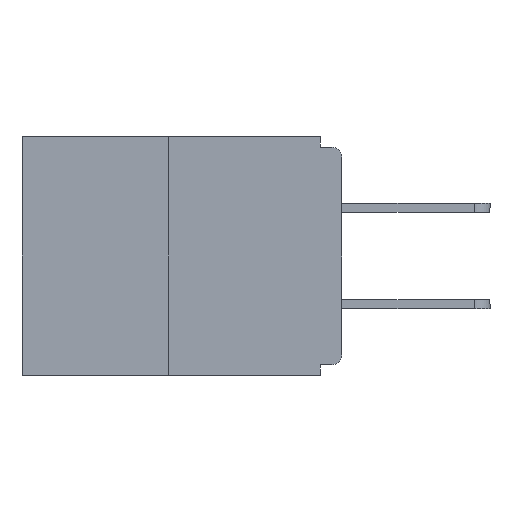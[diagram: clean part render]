
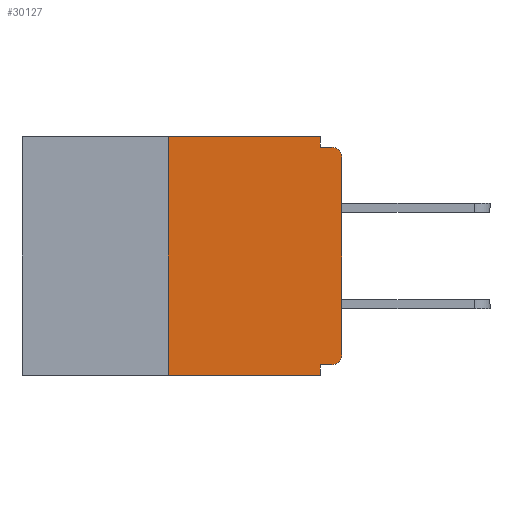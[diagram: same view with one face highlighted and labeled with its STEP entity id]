
A CAD part, left-side view. The second image highlights one B-rep face of the part: STEP entity #30127.
In plain terms, the highlighted planar face has unit normal (-1, 0, 0).
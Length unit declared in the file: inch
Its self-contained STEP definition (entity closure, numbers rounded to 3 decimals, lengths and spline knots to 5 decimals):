
#168 = VECTOR ( 'NONE', #4150, 39.37008 ) ;
#222 = VECTOR ( 'NONE', #31154, 39.37008 ) ;
#537 = CARTESIAN_POINT ( 'NONE',  ( 0., 0.031, -0.328 ) ) ;
#605 = CARTESIAN_POINT ( 'NONE',  ( 0., 0.46, -0.343 ) ) ;
#650 = VECTOR ( 'NONE', #6587, 39.37008 ) ;
#1971 = ORIENTED_EDGE ( 'NONE', *, *, #25293, .F. ) ;
#1997 = LINE ( 'NONE', #8956, #29304 ) ;
#2302 = CARTESIAN_POINT ( 'NONE',  ( 0., 0.031, -0.015 ) ) ;
#2772 = CIRCLE ( 'NONE', #5898, 0.015 ) ;
#2924 = VERTEX_POINT ( 'NONE', #2302 ) ;
#3067 = EDGE_CURVE ( 'NONE', #20193, #16361, #24123, .T. ) ;
#3226 = VERTEX_POINT ( 'NONE', #30207 ) ;
#3488 = DIRECTION ( 'NONE',  ( 0., 0., -1. ) ) ;
#3529 = ORIENTED_EDGE ( 'NONE', *, *, #19720, .F. ) ;
#4104 = CARTESIAN_POINT ( 'NONE',  ( 0., 0.015, -0.015 ) ) ;
#4138 = ORIENTED_EDGE ( 'NONE', *, *, #25420, .F. ) ;
#4150 = DIRECTION ( 'NONE',  ( 0., 0., -1. ) ) ;
#4496 = CARTESIAN_POINT ( 'NONE',  ( 0., 0.25, 0. ) ) ;
#5302 = FACE_OUTER_BOUND ( 'NONE', #24716, .T. ) ;
#5515 = CIRCLE ( 'NONE', #29369, 0.015 ) ;
#5898 = AXIS2_PLACEMENT_3D ( 'NONE', #20658, #10736, #28090 ) ;
#6432 = DIRECTION ( 'NONE',  ( 0., 0., 1. ) ) ;
#6587 = DIRECTION ( 'NONE',  ( 0., 0., 1. ) ) ;
#6754 = CARTESIAN_POINT ( 'NONE',  ( 0., 0.031, 0. ) ) ;
#6783 = DIRECTION ( 'NONE',  ( 1., 0., 0. ) ) ;
#7026 = CARTESIAN_POINT ( 'NONE',  ( 0., 0., 0. ) ) ;
#7106 = LINE ( 'NONE', #7026, #650 ) ;
#7567 = CARTESIAN_POINT ( 'NONE',  ( 0., 0.46, 0. ) ) ;
#7855 = DIRECTION ( 'NONE',  ( 0., -1., 0. ) ) ;
#8956 = CARTESIAN_POINT ( 'NONE',  ( 0., 0.25, 0. ) ) ;
#9000 = CARTESIAN_POINT ( 'NONE',  ( 0., 0.031, -0.343 ) ) ;
#9002 = ORIENTED_EDGE ( 'NONE', *, *, #12672, .F. ) ;
#9441 = CARTESIAN_POINT ( 'NONE',  ( 0., 0., -0.015 ) ) ;
#9682 = ORIENTED_EDGE ( 'NONE', *, *, #10972, .T. ) ;
#10441 = CARTESIAN_POINT ( 'NONE',  ( 0., 0., -0.313 ) ) ;
#10736 = DIRECTION ( 'NONE',  ( -1., 0., 0. ) ) ;
#10972 = EDGE_CURVE ( 'NONE', #27617, #27772, #20453, .T. ) ;
#11623 = DIRECTION ( 'NONE',  ( 0., 0., -1. ) ) ;
#11627 = LINE ( 'NONE', #11649, #30211 ) ;
#11649 = CARTESIAN_POINT ( 'NONE',  ( 0., 0., -0.328 ) ) ;
#11760 = ORIENTED_EDGE ( 'NONE', *, *, #13190, .T. ) ;
#11804 = DIRECTION ( 'NONE',  ( 0., 0., -1. ) ) ;
#12622 = EDGE_CURVE ( 'NONE', #27967, #26005, #7106, .T. ) ;
#12672 = EDGE_CURVE ( 'NONE', #3226, #13007, #11627, .T. ) ;
#13007 = VERTEX_POINT ( 'NONE', #537 ) ;
#13190 = EDGE_CURVE ( 'NONE', #3226, #27967, #5515, .T. ) ;
#14315 = PLANE ( 'NONE',  #19232 ) ;
#15359 = LINE ( 'NONE', #9000, #168 ) ;
#15463 = DIRECTION ( 'NONE',  ( 0., -1., 0. ) ) ;
#15719 = DIRECTION ( 'NONE',  ( -1., 0., 0. ) ) ;
#16305 = CARTESIAN_POINT ( 'NONE',  ( 0., 0., -0.03 ) ) ;
#16361 = VERTEX_POINT ( 'NONE', #20417 ) ;
#16987 = ORIENTED_EDGE ( 'NONE', *, *, #3067, .F. ) ;
#17142 = CARTESIAN_POINT ( 'NONE',  ( 0., 0.031, -0.343 ) ) ;
#17616 = EDGE_CURVE ( 'NONE', #2924, #23178, #30517, .T. ) ;
#18565 = ORIENTED_EDGE ( 'NONE', *, *, #17616, .F. ) ;
#18807 = LINE ( 'NONE', #6754, #19555 ) ;
#19232 = AXIS2_PLACEMENT_3D ( 'NONE', #26232, #6783, #11623 ) ;
#19555 = VECTOR ( 'NONE', #11804, 39.37008 ) ;
#19629 = EDGE_CURVE ( 'NONE', #26005, #23178, #2772, .T. ) ;
#19720 = EDGE_CURVE ( 'NONE', #27617, #20193, #1997, .T. ) ;
#20193 = VERTEX_POINT ( 'NONE', #4496 ) ;
#20360 = CARTESIAN_POINT ( 'NONE',  ( 0., 0.015, -0.313 ) ) ;
#20417 = CARTESIAN_POINT ( 'NONE',  ( 0., 0.031, 0. ) ) ;
#20453 = LINE ( 'NONE', #605, #31016 ) ;
#20658 = CARTESIAN_POINT ( 'NONE',  ( 0., 0.015, -0.03 ) ) ;
#20938 = CARTESIAN_POINT ( 'NONE',  ( 0., 0.25, -0.343 ) ) ;
#22091 = ORIENTED_EDGE ( 'NONE', *, *, #12622, .T. ) ;
#23178 = VERTEX_POINT ( 'NONE', #4104 ) ;
#24123 = LINE ( 'NONE', #7567, #25683 ) ;
#24716 = EDGE_LOOP ( 'NONE', ( #16987, #3529, #9682, #4138, #9002, #11760, #22091, #30137, #18565, #1971 ) ) ;
#25293 = EDGE_CURVE ( 'NONE', #16361, #2924, #18807, .T. ) ;
#25420 = EDGE_CURVE ( 'NONE', #13007, #27772, #15359, .T. ) ;
#25683 = VECTOR ( 'NONE', #7855, 39.37008 ) ;
#26005 = VERTEX_POINT ( 'NONE', #16305 ) ;
#26232 = CARTESIAN_POINT ( 'NONE',  ( 0., 0.46, 0. ) ) ;
#26258 = DIRECTION ( 'NONE',  ( 0., 1., 0. ) ) ;
#27617 = VERTEX_POINT ( 'NONE', #20938 ) ;
#27772 = VERTEX_POINT ( 'NONE', #17142 ) ;
#27967 = VERTEX_POINT ( 'NONE', #10441 ) ;
#28090 = DIRECTION ( 'NONE',  ( 0., 0., -1. ) ) ;
#29304 = VECTOR ( 'NONE', #6432, 39.37008 ) ;
#29369 = AXIS2_PLACEMENT_3D ( 'NONE', #20360, #15719, #3488 ) ;
#30127 = ADVANCED_FACE ( 'NONE', ( #5302 ), #14315, .F. ) ;
#30137 = ORIENTED_EDGE ( 'NONE', *, *, #19629, .T. ) ;
#30207 = CARTESIAN_POINT ( 'NONE',  ( 0., 0.015, -0.328 ) ) ;
#30211 = VECTOR ( 'NONE', #26258, 39.37008 ) ;
#30517 = LINE ( 'NONE', #9441, #222 ) ;
#31016 = VECTOR ( 'NONE', #15463, 39.37008 ) ;
#31154 = DIRECTION ( 'NONE',  ( 0., -1., 0. ) ) ;
